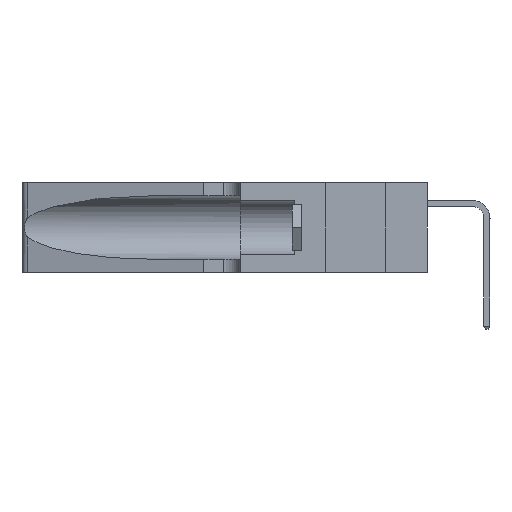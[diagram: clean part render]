
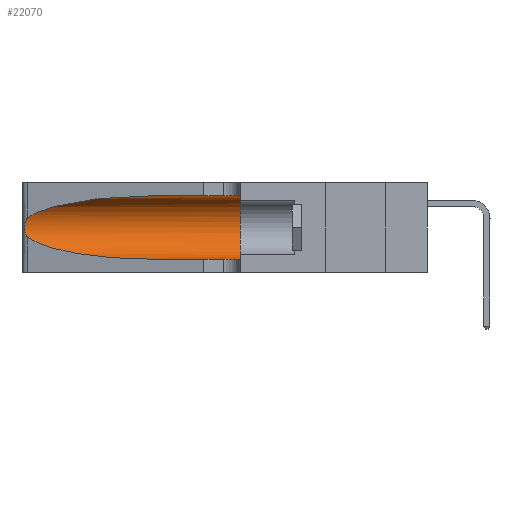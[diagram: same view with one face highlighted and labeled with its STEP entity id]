
A CAD part, left-side view. The second image highlights one B-rep face of the part: STEP entity #22070.
In plain terms, the highlighted cylindrical face has radius 3.308 mm (diameter 6.617 mm), a partial arc.
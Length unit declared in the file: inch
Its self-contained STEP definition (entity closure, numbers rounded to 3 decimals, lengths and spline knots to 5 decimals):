
#19 = CARTESIAN_POINT ( 'NONE',  ( 0.25787, 1.23484, 0.2124 ) ) ;
#420 = CARTESIAN_POINT ( 'NONE',  ( 0.25487, 1.22718, 0.14631 ) ) ;
#736 = EDGE_CURVE ( 'NONE', #22650, #23523, #18525, .T. ) ;
#822 = VECTOR ( 'NONE', #18532, 39.37008 ) ;
#840 = CARTESIAN_POINT ( 'NONE',  ( 0.1305, 0.35, 0.185 ) ) ;
#1040 = CYLINDRICAL_SURFACE ( 'NONE', #22033, 0.13025 ) ;
#1231 = CARTESIAN_POINT ( 'NONE',  ( 0.1305, 1.61858, 0.31525 ) ) ;
#2087 = CARTESIAN_POINT ( 'NONE',  ( 0.26018, 1.23835, 0.19895 ) ) ;
#2929 = DIRECTION ( 'NONE',  ( 0., 0., 1. ) ) ;
#3757 = EDGE_CURVE ( 'NONE', #18993, #26071, #15303, .T. ) ;
#4072 = EDGE_CURVE ( 'NONE', #25714, #19084, #6354, .T. ) ;
#4078 = CARTESIAN_POINT ( 'NONE',  ( 0.25555, 1.22994, 0.2215 ) ) ;
#4174 = CARTESIAN_POINT ( 'NONE',  ( 0.26075, 1.23896, 0.178 ) ) ;
#4563 = CARTESIAN_POINT ( 'NONE',  ( 0.18966, 0.96281, 0.31525 ) ) ;
#5010 = AXIS2_PLACEMENT_3D ( 'NONE', #840, #15208, #2929 ) ;
#5166 =( BOUNDED_CURVE ( )  B_SPLINE_CURVE ( 3, ( #6180, #14384, #6263, #20547 ),
 .UNSPECIFIED., .F., .F. ) 
 B_SPLINE_CURVE_WITH_KNOTS ( ( 4, 4 ),
 ( 3.44316, 4.71239 ),
 .UNSPECIFIED. ) 
 CURVE ( )  GEOMETRIC_REPRESENTATION_ITEM ( )  RATIONAL_B_SPLINE_CURVE ( ( 1., 0.87, 0.87, 1. ) ) 
 REPRESENTATION_ITEM ( '' )  );
#5426 = DIRECTION ( 'NONE',  ( 0., -1., 0. ) ) ;
#5930 = CIRCLE ( 'NONE', #5010, 0.13025 ) ;
#6119 = EDGE_CURVE ( 'NONE', #26071, #19084, #5930, .T. ) ;
#6180 = CARTESIAN_POINT ( 'NONE',  ( 0.25487, 1.22718, 0.14631 ) ) ;
#6227 = DIRECTION ( 'NONE',  ( 0., -1., 0. ) ) ;
#6263 = CARTESIAN_POINT ( 'NONE',  ( 0.18966, 0.96281, 0.05475 ) ) ;
#6276 = CARTESIAN_POINT ( 'NONE',  ( 0.25856, 1.23593, 0.16098 ) ) ;
#6354 = LINE ( 'NONE', #16492, #822 ) ;
#7201 = FACE_OUTER_BOUND ( 'NONE', #24318, .T. ) ;
#8315 = CARTESIAN_POINT ( 'NONE',  ( 0.25639, 1.23186, 0.15144 ) ) ;
#8994 = ORIENTED_EDGE ( 'NONE', *, *, #3757, .F. ) ;
#9183 = CARTESIAN_POINT ( 'NONE',  ( 0.1305, 0.35, 0.31525 ) ) ;
#10121 = EDGE_CURVE ( 'NONE', #23523, #25714, #5166, .T. ) ;
#10307 = CARTESIAN_POINT ( 'NONE',  ( 0.25639, 1.23184, 0.21858 ) ) ;
#10387 = CARTESIAN_POINT ( 'NONE',  ( 0.25487, 1.22718, 0.14631 ) ) ;
#11778 = ORIENTED_EDGE ( 'NONE', *, *, #736, .T. ) ;
#11953 = ORIENTED_EDGE ( 'NONE', *, *, #13970, .T. ) ;
#12313 = CARTESIAN_POINT ( 'NONE',  ( 0.25487, 1.22718, 0.22369 ) ) ;
#12773 = CARTESIAN_POINT ( 'NONE',  ( 0.25487, 1.22718, 0.22369 ) ) ;
#13970 = EDGE_CURVE ( 'NONE', #18993, #22650, #20447, .T. ) ;
#14343 = CARTESIAN_POINT ( 'NONE',  ( 0.1305, 1.61858, 0.185 ) ) ;
#14384 = CARTESIAN_POINT ( 'NONE',  ( 0.2373, 1.15595, 0.08982 ) ) ;
#14393 = CARTESIAN_POINT ( 'NONE',  ( 0.25854, 1.2359, 0.20912 ) ) ;
#14401 = CARTESIAN_POINT ( 'NONE',  ( 0.25487, 1.22718, 0.22369 ) ) ;
#15208 = DIRECTION ( 'NONE',  ( 0., 1., 0. ) ) ;
#15303 = LINE ( 'NONE', #1231, #24899 ) ;
#16400 = DIRECTION ( 'NONE',  ( 0., 0., -1. ) ) ;
#16452 = CARTESIAN_POINT ( 'NONE',  ( 0.26075, 1.23896, 0.19203 ) ) ;
#16492 = CARTESIAN_POINT ( 'NONE',  ( 0.1305, 1.61858, 0.05475 ) ) ;
#17898 = CARTESIAN_POINT ( 'NONE',  ( 0.1305, 0.35, 0.05475 ) ) ;
#18199 = ORIENTED_EDGE ( 'NONE', *, *, #4072, .T. ) ;
#18498 = CARTESIAN_POINT ( 'NONE',  ( 0.26017, 1.23833, 0.17102 ) ) ;
#18525 = B_SPLINE_CURVE_WITH_KNOTS ( 'NONE', 3,
 ( #12313, #4078, #10307, #19, #14393, #2087, #16452, #4174, #18498, #6276, #20560, #8315, #22587, #10387 ),
 .UNSPECIFIED., .F., .F.,
 ( 4, 2, 2, 2, 2, 2, 4 ),
 ( 0., 0.00027, 0.00053, 0.00107, 0.0016, 0.00187, 0.00214 ),
 .UNSPECIFIED. ) ;
#18532 = DIRECTION ( 'NONE',  ( 0., -1., 0. ) ) ;
#18993 = VERTEX_POINT ( 'NONE', #21379 ) ;
#19084 = VERTEX_POINT ( 'NONE', #17898 ) ;
#20291 = CARTESIAN_POINT ( 'NONE',  ( 0.1305, 0.72297, 0.05475 ) ) ;
#20447 =( BOUNDED_CURVE ( )  B_SPLINE_CURVE ( 3, ( #22953, #4563, #25034, #12773 ),
 .UNSPECIFIED., .F., .T. ) 
 B_SPLINE_CURVE_WITH_KNOTS ( ( 4, 4 ),
 ( 1.5708, 2.84003 ),
 .UNSPECIFIED. ) 
 CURVE ( )  GEOMETRIC_REPRESENTATION_ITEM ( )  RATIONAL_B_SPLINE_CURVE ( ( 1., 0.87, 0.87, 1. ) ) 
 REPRESENTATION_ITEM ( '' )  );
#20547 = CARTESIAN_POINT ( 'NONE',  ( 0.1305, 0.72297, 0.05475 ) ) ;
#20560 = CARTESIAN_POINT ( 'NONE',  ( 0.25789, 1.23486, 0.15765 ) ) ;
#21379 = CARTESIAN_POINT ( 'NONE',  ( 0.1305, 0.72297, 0.31525 ) ) ;
#22033 = AXIS2_PLACEMENT_3D ( 'NONE', #14343, #6227, #16400 ) ;
#22070 = ADVANCED_FACE ( 'NONE', ( #7201 ), #1040, .F. ) ;
#22587 = CARTESIAN_POINT ( 'NONE',  ( 0.25555, 1.22993, 0.14849 ) ) ;
#22650 = VERTEX_POINT ( 'NONE', #14401 ) ;
#22879 = ORIENTED_EDGE ( 'NONE', *, *, #10121, .T. ) ;
#22953 = CARTESIAN_POINT ( 'NONE',  ( 0.1305, 0.72297, 0.31525 ) ) ;
#23523 = VERTEX_POINT ( 'NONE', #420 ) ;
#24318 = EDGE_LOOP ( 'NONE', ( #11953, #11778, #22879, #18199, #24732, #8994 ) ) ;
#24732 = ORIENTED_EDGE ( 'NONE', *, *, #6119, .F. ) ;
#24899 = VECTOR ( 'NONE', #5426, 39.37008 ) ;
#25034 = CARTESIAN_POINT ( 'NONE',  ( 0.2373, 1.15595, 0.28018 ) ) ;
#25714 = VERTEX_POINT ( 'NONE', #20291 ) ;
#26071 = VERTEX_POINT ( 'NONE', #9183 ) ;
